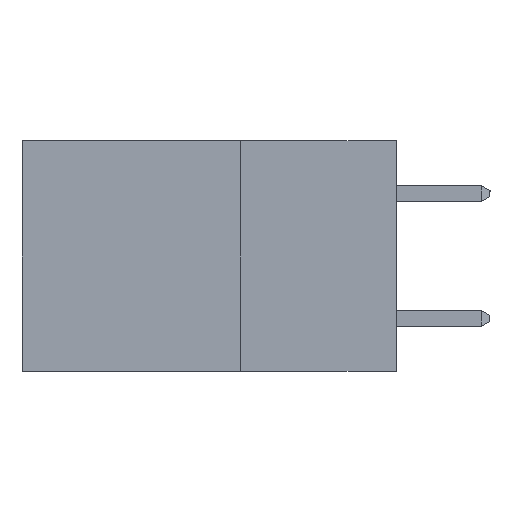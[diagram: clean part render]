
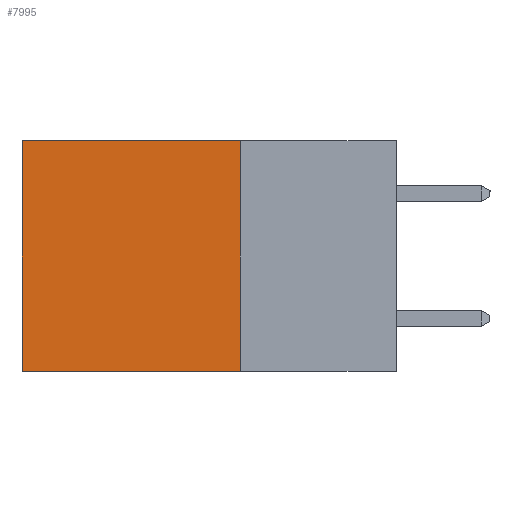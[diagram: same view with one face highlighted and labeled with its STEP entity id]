
A CAD part, left-side view. The second image highlights one B-rep face of the part: STEP entity #7995.
In plain terms, the highlighted planar face has unit normal (-1, 0, 0).
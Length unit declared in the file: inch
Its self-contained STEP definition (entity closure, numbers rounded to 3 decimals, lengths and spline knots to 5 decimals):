
#319 = VERTEX_POINT ( 'NONE', #9395 ) ;
#409 = VECTOR ( 'NONE', #6283, 39.37008 ) ;
#672 = VERTEX_POINT ( 'NONE', #4377 ) ;
#762 = FACE_OUTER_BOUND ( 'NONE', #6794, .T. ) ;
#810 = DIRECTION ( 'NONE',  ( 0., 1., 0. ) ) ;
#877 = CARTESIAN_POINT ( 'NONE',  ( 0.2615, 0.25, -0.37 ) ) ;
#1591 = VECTOR ( 'NONE', #6630, 39.37008 ) ;
#1944 = LINE ( 'NONE', #7929, #409 ) ;
#2713 = EDGE_CURVE ( 'NONE', #5203, #4141, #1944, .T. ) ;
#3231 = PLANE ( 'NONE',  #7456 ) ;
#3238 = CARTESIAN_POINT ( 'NONE',  ( 0.2615, 0.25, -0.37 ) ) ;
#3389 = ORIENTED_EDGE ( 'NONE', *, *, #2713, .F. ) ;
#4141 = VERTEX_POINT ( 'NONE', #5830 ) ;
#4377 = CARTESIAN_POINT ( 'NONE',  ( 0.2615, 0.6, 0. ) ) ;
#5203 = VERTEX_POINT ( 'NONE', #5652 ) ;
#5634 = EDGE_CURVE ( 'NONE', #672, #319, #7276, .T. ) ;
#5652 = CARTESIAN_POINT ( 'NONE',  ( 0.2615, 0.25, 0. ) ) ;
#5825 = VECTOR ( 'NONE', #9075, 39.37008 ) ;
#5830 = CARTESIAN_POINT ( 'NONE',  ( 0.2615, 0.25, -0.37 ) ) ;
#5836 = DIRECTION ( 'NONE',  ( 1., 0., 0. ) ) ;
#5946 = DIRECTION ( 'NONE',  ( 0., 0., -1. ) ) ;
#6283 = DIRECTION ( 'NONE',  ( 0., 0., -1. ) ) ;
#6630 = DIRECTION ( 'NONE',  ( 0., 1., 0. ) ) ;
#6794 = EDGE_LOOP ( 'NONE', ( #10902, #7934, #3389, #9133 ) ) ;
#6835 = EDGE_CURVE ( 'NONE', #5203, #672, #8518, .T. ) ;
#6922 = VECTOR ( 'NONE', #810, 39.37008 ) ;
#7276 = LINE ( 'NONE', #9127, #5825 ) ;
#7456 = AXIS2_PLACEMENT_3D ( 'NONE', #877, #5836, #5946 ) ;
#7929 = CARTESIAN_POINT ( 'NONE',  ( 0.2615, 0.25, -0.37 ) ) ;
#7934 = ORIENTED_EDGE ( 'NONE', *, *, #9251, .F. ) ;
#7995 = ADVANCED_FACE ( 'NONE', ( #762 ), #3231, .F. ) ;
#8271 = LINE ( 'NONE', #3238, #1591 ) ;
#8518 = LINE ( 'NONE', #9585, #6922 ) ;
#9075 = DIRECTION ( 'NONE',  ( 0., 0., -1. ) ) ;
#9127 = CARTESIAN_POINT ( 'NONE',  ( 0.2615, 0.6, -0.37 ) ) ;
#9133 = ORIENTED_EDGE ( 'NONE', *, *, #6835, .T. ) ;
#9251 = EDGE_CURVE ( 'NONE', #4141, #319, #8271, .T. ) ;
#9395 = CARTESIAN_POINT ( 'NONE',  ( 0.2615, 0.6, -0.37 ) ) ;
#9585 = CARTESIAN_POINT ( 'NONE',  ( 0.2615, 0.25, 0. ) ) ;
#10902 = ORIENTED_EDGE ( 'NONE', *, *, #5634, .T. ) ;
